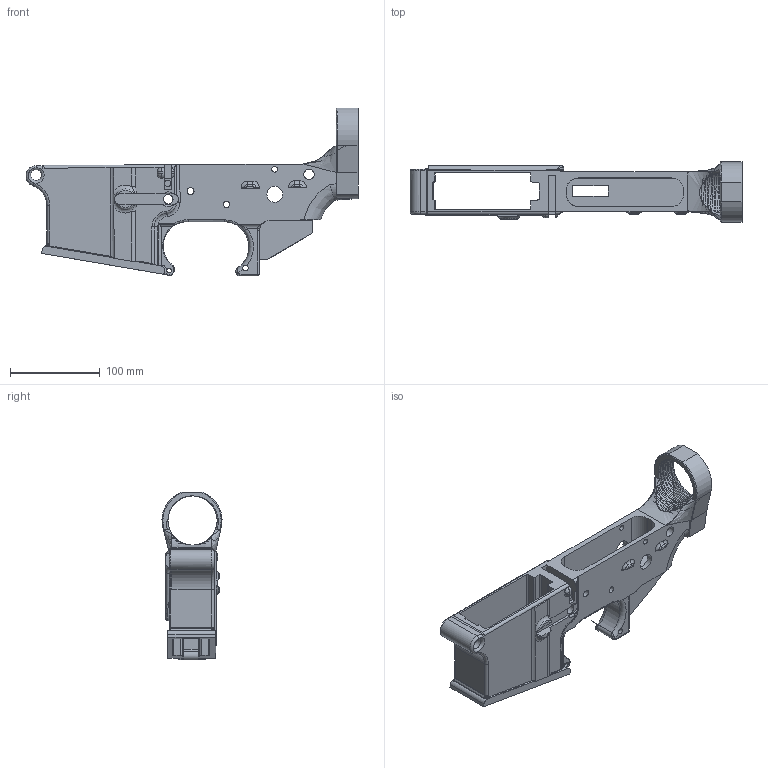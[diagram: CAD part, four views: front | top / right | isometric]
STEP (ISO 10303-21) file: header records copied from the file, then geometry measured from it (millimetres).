
FILE_DESCRIPTION(/* description */ (''),/* implementation_level */ '2;1');
FILE_NAME(/* name */ '5fb32b0469fc831247e11469',/* time_stamp */ '2020-11-17T01:44:37+00:00',/* author */ (''),/* organization */ (''),/* preprocessor_version */ 'ST-DEVELOPER v16.7',/* originating_system */ $,/* authorisation */ $);
FILE_SCHEMA (('AUTOMOTIVE_DESIGN {1 0 10303 214 3 1 1}'));
Length unit declared in the file: metre
Products named in the file (6): Curve 1; Part 5; Part 4; Part 3; Part 2; Part 1
Bounding box: 370.46 x 66.99 x 187.45 mm (x, y, z)
Volume: 730715.8 mm3; surface area: 194353.4 mm2
Topology: 5 solids, 5 shells, 412 faces, 1108 edges, 697 vertices
Faces by surface type: cylinder 151, plane 124, bspline 84, torus 49, sphere 4
Full cylindrical faces by diameter (mm): 5.181 x2, 6.068 x1, 6.197 x2, 6.999 x2, 7.806 x1, 7.812 x2, 10.54 x1, 11.586 x1, 12.288 x1, 17.757 x2
Entity records: 20400 total; most frequent: CARTESIAN_POINT 10781, ORIENTED_EDGE 2134, DIRECTION 1741, EDGE_CURVE 1067, VERTEX_POINT 681, AXIS2_PLACEMENT_3D 658, EDGE_LOOP 464, FACE_BOUND 464
